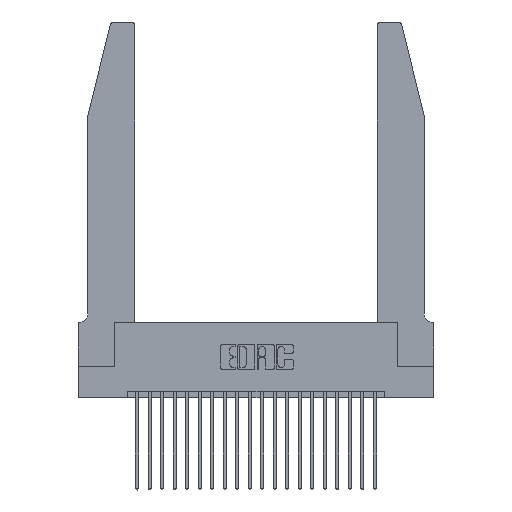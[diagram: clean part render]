
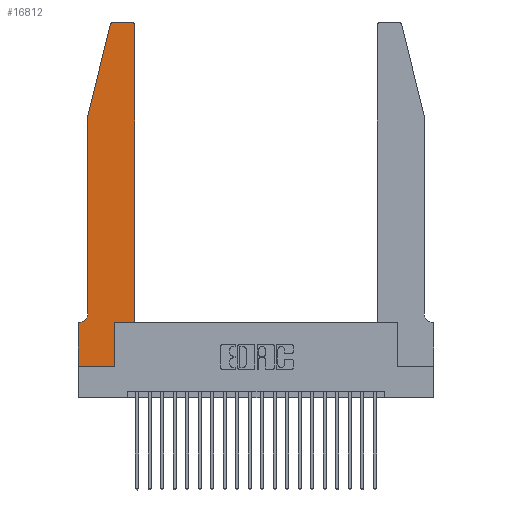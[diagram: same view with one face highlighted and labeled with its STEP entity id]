
A CAD part, top view. The second image highlights one B-rep face of the part: STEP entity #16812.
In plain terms, the highlighted planar face has unit normal (0, 0, 1).
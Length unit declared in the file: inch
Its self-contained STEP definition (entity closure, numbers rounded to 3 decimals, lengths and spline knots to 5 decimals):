
#445 = LINE ( 'NONE', #7094, #15152 ) ;
#467 = ORIENTED_EDGE ( 'NONE', *, *, #10432, .T. ) ;
#504 = EDGE_CURVE ( 'NONE', #21820, #2542, #15710, .T. ) ;
#1164 = VERTEX_POINT ( 'NONE', #4912 ) ;
#1249 = EDGE_CURVE ( 'NONE', #19774, #2025, #18480, .T. ) ;
#1280 = VECTOR ( 'NONE', #3779, 39.37008 ) ;
#1779 = DIRECTION ( 'NONE',  ( 0., -1., 0. ) ) ;
#2025 = VERTEX_POINT ( 'NONE', #7149 ) ;
#2106 = CARTESIAN_POINT ( 'NONE',  ( 0.0055, 0.35, 0.37 ) ) ;
#2391 = VECTOR ( 'NONE', #15291, 39.37008 ) ;
#2424 = LINE ( 'NONE', #19240, #13455 ) ;
#2542 = VERTEX_POINT ( 'NONE', #8967 ) ;
#2790 = CARTESIAN_POINT ( 'NONE',  ( 0.4505, 0.35, 0.37 ) ) ;
#3211 = VECTOR ( 'NONE', #11082, 39.37008 ) ;
#3779 = DIRECTION ( 'NONE',  ( 1., 0., 0. ) ) ;
#3856 = VERTEX_POINT ( 'NONE', #21422 ) ;
#4372 = CIRCLE ( 'NONE', #21671, 0.07 ) ;
#4449 = EDGE_CURVE ( 'NONE', #12778, #21820, #20922, .T. ) ;
#4469 = CARTESIAN_POINT ( 'NONE',  ( 0., 0., 0.37 ) ) ;
#4912 = CARTESIAN_POINT ( 'NONE',  ( 0.0755, 2., 0.37 ) ) ;
#5257 = LINE ( 'NONE', #21882, #1280 ) ;
#5305 = DIRECTION ( 'NONE',  ( 0., 0., -1. ) ) ;
#5781 = VERTEX_POINT ( 'NONE', #8992 ) ;
#5952 = ORIENTED_EDGE ( 'NONE', *, *, #17738, .T. ) ;
#6072 = LINE ( 'NONE', #7527, #3211 ) ;
#6309 = EDGE_LOOP ( 'NONE', ( #11576, #467, #22478, #21654, #5952, #21935, #16584, #17776, #15200, #20857, #20045, #22334 ) ) ;
#6602 = DIRECTION ( 'NONE',  ( 0., 1., 0. ) ) ;
#6611 = CARTESIAN_POINT ( 'NONE',  ( 0., 0., 0.37 ) ) ;
#7049 = EDGE_CURVE ( 'NONE', #18756, #20778, #5257, .T. ) ;
#7094 = CARTESIAN_POINT ( 'NONE',  ( 0.0755, 2., 0.37 ) ) ;
#7125 = DIRECTION ( 'NONE',  ( -1., 0., 0. ) ) ;
#7149 = CARTESIAN_POINT ( 'NONE',  ( 0., 0.35, 0.37 ) ) ;
#7527 = CARTESIAN_POINT ( 'NONE',  ( 0.4505, 0.35, 0.37 ) ) ;
#7866 = CARTESIAN_POINT ( 'NONE',  ( 0.4205, 2.75, 0.37 ) ) ;
#7953 = CIRCLE ( 'NONE', #19684, 0.03 ) ;
#8580 = EDGE_CURVE ( 'NONE', #21548, #12778, #6072, .T. ) ;
#8745 = CARTESIAN_POINT ( 'NONE',  ( 0.4505, 0.35, 0.37 ) ) ;
#8751 = LINE ( 'NONE', #20435, #11021 ) ;
#8896 = CARTESIAN_POINT ( 'NONE',  ( 0.4205, 2.72, 0.37 ) ) ;
#8967 = CARTESIAN_POINT ( 'NONE',  ( 0.284, 2.75, 0.37 ) ) ;
#8992 = CARTESIAN_POINT ( 'NONE',  ( 0.25487, 2.72718, 0.37 ) ) ;
#9060 = DIRECTION ( 'NONE',  ( -1., 0., 0. ) ) ;
#9493 = DIRECTION ( 'NONE',  ( 1., 0., 0. ) ) ;
#9700 = DIRECTION ( 'NONE',  ( -1., 0., 0. ) ) ;
#9980 = AXIS2_PLACEMENT_3D ( 'NONE', #14313, #21378, #10845 ) ;
#10432 = EDGE_CURVE ( 'NONE', #2542, #5781, #7953, .T. ) ;
#10691 = PLANE ( 'NONE',  #9980 ) ;
#10845 = DIRECTION ( 'NONE',  ( 1., 0., 0. ) ) ;
#10875 = FACE_OUTER_BOUND ( 'NONE', #6309, .T. ) ;
#11021 = VECTOR ( 'NONE', #11321, 39.37008 ) ;
#11082 = DIRECTION ( 'NONE',  ( 0., 1., 0. ) ) ;
#11321 = DIRECTION ( 'NONE',  ( -0.239, -0.971, 0. ) ) ;
#11576 = ORIENTED_EDGE ( 'NONE', *, *, #504, .T. ) ;
#12255 = EDGE_CURVE ( 'NONE', #5781, #1164, #8751, .T. ) ;
#12492 = LINE ( 'NONE', #6611, #17594 ) ;
#12778 = VERTEX_POINT ( 'NONE', #18574 ) ;
#13455 = VECTOR ( 'NONE', #6602, 39.37008 ) ;
#13658 = DIRECTION ( 'NONE',  ( 1., 0., 0. ) ) ;
#13739 = DIRECTION ( 'NONE',  ( 0., 0., 1. ) ) ;
#14285 = VECTOR ( 'NONE', #9060, 39.37008 ) ;
#14313 = CARTESIAN_POINT ( 'NONE',  ( 0., 0.35, 0.37 ) ) ;
#14445 = CARTESIAN_POINT ( 'NONE',  ( 0.2865, 0.35, 0.37 ) ) ;
#14509 = EDGE_CURVE ( 'NONE', #1164, #3856, #445, .T. ) ;
#15152 = VECTOR ( 'NONE', #1779, 39.37008 ) ;
#15200 = ORIENTED_EDGE ( 'NONE', *, *, #22688, .T. ) ;
#15291 = DIRECTION ( 'NONE',  ( 1., 0., 0. ) ) ;
#15416 = LINE ( 'NONE', #2790, #2391 ) ;
#15710 = LINE ( 'NONE', #16403, #14285 ) ;
#16240 = VECTOR ( 'NONE', #9700, 39.37008 ) ;
#16403 = CARTESIAN_POINT ( 'NONE',  ( 0.2605, 2.75, 0.37 ) ) ;
#16566 = EDGE_CURVE ( 'NONE', #21690, #21548, #15416, .T. ) ;
#16584 = ORIENTED_EDGE ( 'NONE', *, *, #18970, .T. ) ;
#16812 = ADVANCED_FACE ( 'NONE', ( #10875 ), #10691, .T. ) ;
#16916 = DIRECTION ( 'NONE',  ( 0., 0., 1. ) ) ;
#17594 = VECTOR ( 'NONE', #19321, 39.37008 ) ;
#17738 = EDGE_CURVE ( 'NONE', #3856, #19774, #4372, .T. ) ;
#17776 = ORIENTED_EDGE ( 'NONE', *, *, #7049, .T. ) ;
#17956 = AXIS2_PLACEMENT_3D ( 'NONE', #8896, #13739, #13658 ) ;
#18173 = CARTESIAN_POINT ( 'NONE',  ( 0.0055, 0.42, 0.37 ) ) ;
#18480 = LINE ( 'NONE', #21125, #16240 ) ;
#18574 = CARTESIAN_POINT ( 'NONE',  ( 0.4505, 2.72, 0.37 ) ) ;
#18756 = VERTEX_POINT ( 'NONE', #4469 ) ;
#18970 = EDGE_CURVE ( 'NONE', #2025, #18756, #12492, .T. ) ;
#19240 = CARTESIAN_POINT ( 'NONE',  ( 0.2865, 0.35, 0.37 ) ) ;
#19321 = DIRECTION ( 'NONE',  ( 0., -1., 0. ) ) ;
#19684 = AXIS2_PLACEMENT_3D ( 'NONE', #20584, #16916, #9493 ) ;
#19774 = VERTEX_POINT ( 'NONE', #2106 ) ;
#20045 = ORIENTED_EDGE ( 'NONE', *, *, #8580, .T. ) ;
#20435 = CARTESIAN_POINT ( 'NONE',  ( 0.0755, 2., 0.37 ) ) ;
#20584 = CARTESIAN_POINT ( 'NONE',  ( 0.284, 2.72, 0.37 ) ) ;
#20778 = VERTEX_POINT ( 'NONE', #22985 ) ;
#20857 = ORIENTED_EDGE ( 'NONE', *, *, #16566, .T. ) ;
#20922 = CIRCLE ( 'NONE', #17956, 0.03 ) ;
#21125 = CARTESIAN_POINT ( 'NONE',  ( 0.0755, 0.35, 0.37 ) ) ;
#21378 = DIRECTION ( 'NONE',  ( 0., 0., 1. ) ) ;
#21422 = CARTESIAN_POINT ( 'NONE',  ( 0.0755, 0.42, 0.37 ) ) ;
#21548 = VERTEX_POINT ( 'NONE', #8745 ) ;
#21654 = ORIENTED_EDGE ( 'NONE', *, *, #14509, .T. ) ;
#21671 = AXIS2_PLACEMENT_3D ( 'NONE', #18173, #5305, #7125 ) ;
#21690 = VERTEX_POINT ( 'NONE', #14445 ) ;
#21820 = VERTEX_POINT ( 'NONE', #7866 ) ;
#21882 = CARTESIAN_POINT ( 'NONE',  ( 0., 0., 0.37 ) ) ;
#21935 = ORIENTED_EDGE ( 'NONE', *, *, #1249, .T. ) ;
#22334 = ORIENTED_EDGE ( 'NONE', *, *, #4449, .T. ) ;
#22478 = ORIENTED_EDGE ( 'NONE', *, *, #12255, .T. ) ;
#22688 = EDGE_CURVE ( 'NONE', #20778, #21690, #2424, .T. ) ;
#22985 = CARTESIAN_POINT ( 'NONE',  ( 0.2865, 0., 0.37 ) ) ;
